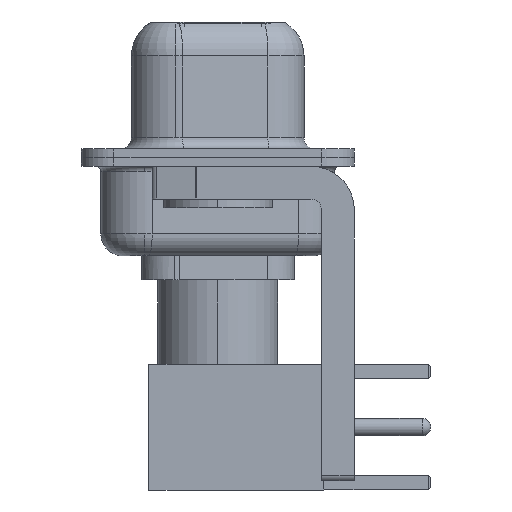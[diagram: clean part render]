
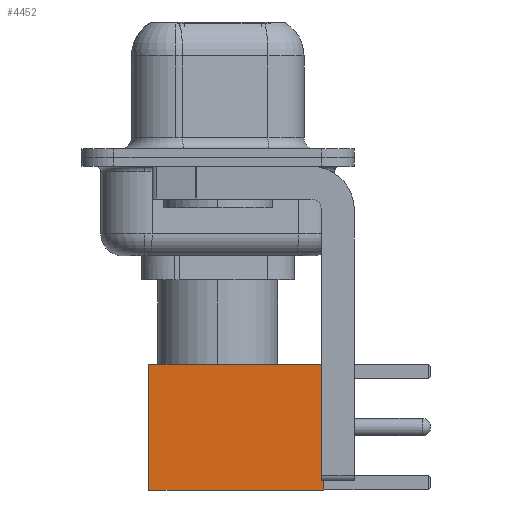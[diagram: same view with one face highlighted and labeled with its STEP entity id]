
A CAD part, left-side view. The second image highlights one B-rep face of the part: STEP entity #4452.
In plain terms, the highlighted face is planar.
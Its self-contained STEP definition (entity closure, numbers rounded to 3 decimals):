
#153 = CARTESIAN_POINT ( 'NONE',  ( 2.875, 2.875, 0. ) ) ;
#1146 = LINE ( 'NONE', #13621, #9305 ) ;
#1396 = EDGE_CURVE ( 'NONE', #4484, #12844, #1146, .T. ) ;
#2091 = LINE ( 'NONE', #5970, #17435 ) ;
#2240 = LINE ( 'NONE', #7511, #13809 ) ;
#2660 = CARTESIAN_POINT ( 'NONE',  ( 2.875, 2.875, 0. ) ) ;
#3280 = DIRECTION ( 'NONE',  ( 0., 0., -1. ) ) ;
#3829 = DIRECTION ( 'NONE',  ( 0., 0., 1. ) ) ;
#4146 = CARTESIAN_POINT ( 'NONE',  ( -2.875, 2.875, 0. ) ) ;
#4452 = ADVANCED_FACE ( 'NONE', ( #8225 ), #9387, .T. ) ;
#4484 = VERTEX_POINT ( 'NONE', #11886 ) ;
#5729 = ORIENTED_EDGE ( 'NONE', *, *, #12534, .T. ) ;
#5970 = CARTESIAN_POINT ( 'NONE',  ( 2.875, 2.875, 0. ) ) ;
#6070 = ORIENTED_EDGE ( 'NONE', *, *, #1396, .F. ) ;
#6475 = VERTEX_POINT ( 'NONE', #4146 ) ;
#6683 = DIRECTION ( 'NONE',  ( 0., 1., 0. ) ) ;
#7511 = CARTESIAN_POINT ( 'NONE',  ( -2.875, 2.875, 0. ) ) ;
#7689 = VERTEX_POINT ( 'NONE', #153 ) ;
#7695 = EDGE_LOOP ( 'NONE', ( #10423, #5729, #13163, #6070 ) ) ;
#8225 = FACE_OUTER_BOUND ( 'NONE', #7695, .T. ) ;
#8988 = EDGE_CURVE ( 'NONE', #4484, #7689, #2091, .T. ) ;
#9305 = VECTOR ( 'NONE', #10742, 1000. ) ;
#9387 = PLANE ( 'NONE',  #13379 ) ;
#10423 = ORIENTED_EDGE ( 'NONE', *, *, #8988, .T. ) ;
#10645 = VECTOR ( 'NONE', #10721, 1000. ) ;
#10721 = DIRECTION ( 'NONE',  ( -1., 0., 0. ) ) ;
#10742 = DIRECTION ( 'NONE',  ( -1., 0., 0. ) ) ;
#10990 = LINE ( 'NONE', #13700, #10645 ) ;
#11886 = CARTESIAN_POINT ( 'NONE',  ( 2.875, 2.875, 8. ) ) ;
#12534 = EDGE_CURVE ( 'NONE', #7689, #6475, #10990, .T. ) ;
#12844 = VERTEX_POINT ( 'NONE', #15208 ) ;
#13163 = ORIENTED_EDGE ( 'NONE', *, *, #13353, .F. ) ;
#13353 = EDGE_CURVE ( 'NONE', #12844, #6475, #2240, .T. ) ;
#13379 = AXIS2_PLACEMENT_3D ( 'NONE', #2660, #6683, #3829 ) ;
#13621 = CARTESIAN_POINT ( 'NONE',  ( 0., 2.875, 8. ) ) ;
#13700 = CARTESIAN_POINT ( 'NONE',  ( 0., 2.875, 0. ) ) ;
#13809 = VECTOR ( 'NONE', #15506, 1000. ) ;
#15208 = CARTESIAN_POINT ( 'NONE',  ( -2.875, 2.875, 8. ) ) ;
#15506 = DIRECTION ( 'NONE',  ( 0., 0., -1. ) ) ;
#17435 = VECTOR ( 'NONE', #3280, 1000. ) ;
